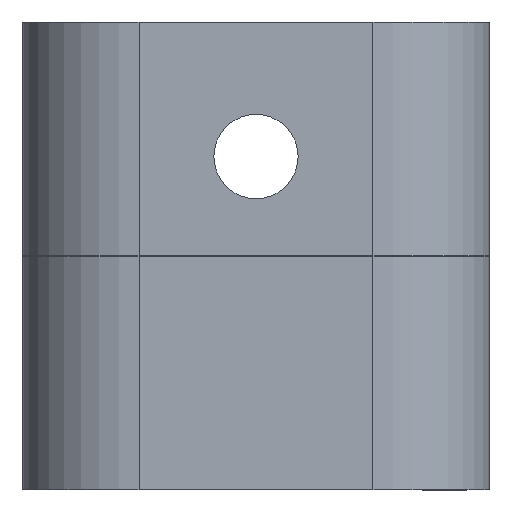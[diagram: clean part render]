
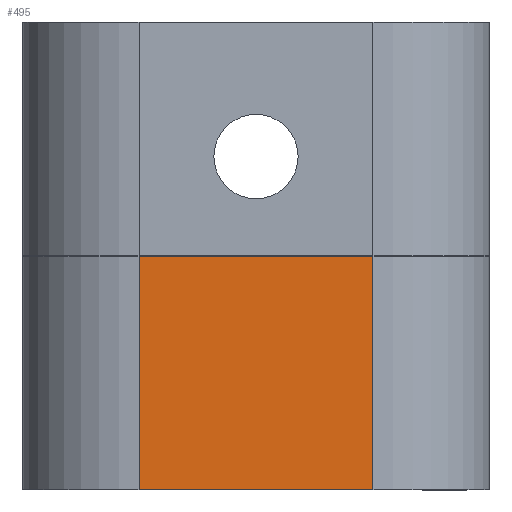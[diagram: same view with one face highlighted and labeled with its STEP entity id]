
A CAD part, left-side view. The second image highlights one B-rep face of the part: STEP entity #495.
In plain terms, the highlighted face is planar.
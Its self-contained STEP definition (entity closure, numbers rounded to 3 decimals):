
#45=PLANE('',#572);
#71=FACE_OUTER_BOUND('',#105,.T.);
#105=EDGE_LOOP('',(#437,#438,#439,#440));
#140=LINE('',#842,#182);
#150=LINE('',#866,#192);
#151=LINE('',#870,#193);
#152=LINE('',#871,#194);
#182=VECTOR('',#690,10.);
#192=VECTOR('',#712,10.);
#193=VECTOR('',#717,10.);
#194=VECTOR('',#718,10.);
#252=VERTEX_POINT('',#839);
#253=VERTEX_POINT('',#841);
#261=VERTEX_POINT('',#865);
#262=VERTEX_POINT('',#869);
#310=EDGE_CURVE('',#253,#252,#140,.T.);
#322=EDGE_CURVE('',#253,#261,#150,.T.);
#324=EDGE_CURVE('',#262,#252,#151,.T.);
#325=EDGE_CURVE('',#262,#261,#152,.T.);
#437=ORIENTED_EDGE('',*,*,#322,.F.);
#438=ORIENTED_EDGE('',*,*,#310,.T.);
#439=ORIENTED_EDGE('',*,*,#324,.F.);
#440=ORIENTED_EDGE('',*,*,#325,.T.);
#495=ADVANCED_FACE('',(#71),#45,.T.);
#572=AXIS2_PLACEMENT_3D('',#868,#715,#716);
#690=DIRECTION('',(-0.707,0.707,0.));
#712=DIRECTION('',(0.,0.,-1.));
#715=DIRECTION('center_axis',(-0.707,-0.707,0.));
#716=DIRECTION('ref_axis',(0.707,-0.707,0.));
#717=DIRECTION('',(0.,0.,1.));
#718=DIRECTION('',(0.707,-0.707,0.));
#839=CARTESIAN_POINT('',(-24.497,-42.426,20.));
#841=CARTESIAN_POINT('',(-17.426,-49.497,20.));
#842=CARTESIAN_POINT('',(-24.497,-42.426,20.));
#865=CARTESIAN_POINT('',(-17.426,-49.497,10.));
#866=CARTESIAN_POINT('',(-17.426,-49.497,17.5));
#868=CARTESIAN_POINT('Origin',(-20.962,-45.962,15.));
#869=CARTESIAN_POINT('',(-24.497,-42.426,10.));
#870=CARTESIAN_POINT('',(-24.497,-42.426,12.5));
#871=CARTESIAN_POINT('',(-17.426,-49.497,10.));
